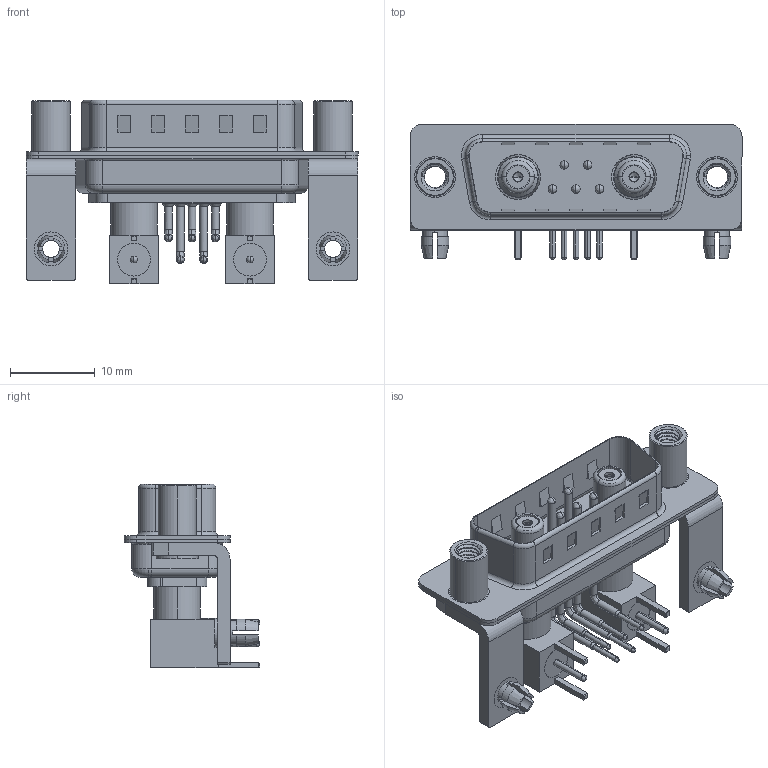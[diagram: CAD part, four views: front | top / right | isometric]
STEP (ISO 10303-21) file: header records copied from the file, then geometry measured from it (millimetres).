
FILE_DESCRIPTION (( 'STEP AP203' ), '1' );
FILE_NAME ('629-7W2-640-5TD.STEP', '2022-05-09T19:22:12', ( '' ), ( '' ), 'SwSTEP 2.0', 'SolidWorks 2020', '' );
FILE_SCHEMA (( 'CONFIG_CONTROL_DESIGN' ));
Length unit declared in the file: millimetre
Products named in the file (18): Insulator Socket 2; 629Combo Shell Front_15 Contacts; 629Combo Housing_7W2; 629-7W2-640-5TD; 629Combo Shell Rear_15 Contacts; Insulator RA Pin; Co-Ax Jack Assy_RA; Socket_RA; Insulator Socket; 629Combo Threaded Standoff_D; 629Combo Contact Row 2; Co-Ax Jack_RA PC Tail; 629Combo Stabilizer Bracket; RA Back Shell; 629Combo Board Lock; Locking Collar; 629Combo Contact Row 1
Assembly tree (30 placements, depth 3):
  629-7W2-640-5TD
    629Combo Housing_7W2
    629Combo Shell Rear_15 Contacts
    629Combo Shell Front_15 Contacts
    629Combo Stabilizer Bracket  x2
    629Combo Board Lock  x2
    629Combo Threaded Standoff_D  x2
    Co-Ax Jack Assy_RA
      Co-Ax Jack_RA PC Tail
      Insulator Socket
      Insulator Socket 2
      Locking Collar
      Socket_RA
      RA Back Shell
      Insulator RA Pin
    Co-Ax Jack Assy_RA
      Co-Ax Jack_RA PC Tail
      Insulator Socket
      Insulator Socket 2
      Locking Collar
      Socket_RA
      RA Back Shell
      Insulator RA Pin
    629Combo Contact Row 1  x2
    629Combo Contact Row 2  x3
Bounding box: 39.2 x 16 x 21.71 mm (x, y, z)
Volume: 2870.7 mm3; surface area: 7918 mm2
Topology: 28 solids, 28 shells, 1384 faces, 3615 edges, 2316 vertices
Faces by surface type: plane 643, cylinder 551, cone 86, torus 62, bspline 38, sphere 4
Entity records: 29214 total; most frequent: CARTESIAN_POINT 7014, DIRECTION 4316, ORIENTED_EDGE 4092, EDGE_CURVE 2046, AXIS2_PLACEMENT_3D 1564, VERTEX_POINT 1316, LINE 1188, VECTOR 1188
